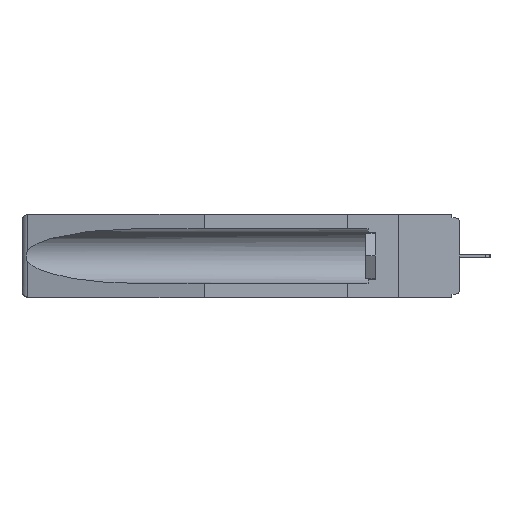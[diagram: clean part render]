
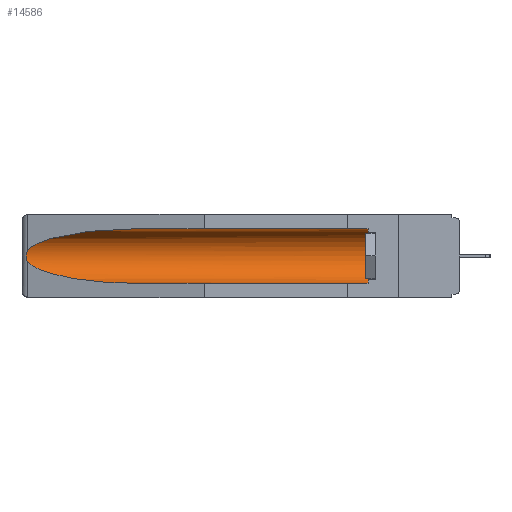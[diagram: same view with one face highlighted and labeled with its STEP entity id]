
A CAD part, left-side view. The second image highlights one B-rep face of the part: STEP entity #14586.
In plain terms, the highlighted cylindrical face has radius 2.857 mm (diameter 5.715 mm), a partial arc.
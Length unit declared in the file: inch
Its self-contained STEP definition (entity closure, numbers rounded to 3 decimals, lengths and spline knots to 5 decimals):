
#298 = EDGE_CURVE ( 'NONE', #9686, #6694, #29425, .T. ) ;
#1093 = AXIS2_PLACEMENT_3D ( 'NONE', #24603, #8456, #6335 ) ;
#1912 = LINE ( 'NONE', #9284, #27571 ) ;
#2595 = AXIS2_PLACEMENT_3D ( 'NONE', #17947, #6588, #8894 ) ;
#3220 = CARTESIAN_POINT ( 'NONE',  ( 0.26597, 1.52961, -0.15275 ) ) ;
#3482 = VERTEX_POINT ( 'NONE', #27198 ) ;
#4576 = CIRCLE ( 'NONE', #2595, 0.1125 ) ;
#4707 =( BOUNDED_CURVE ( )  B_SPLINE_CURVE ( 3, ( #25075, #24777, #6826, #13353 ),
 .UNSPECIFIED., .F., .F. ) 
 B_SPLINE_CURVE_WITH_KNOTS ( ( 4, 4 ),
 ( 4.71239, 6.08839 ),
 .UNSPECIFIED. ) 
 CURVE ( )  GEOMETRIC_REPRESENTATION_ITEM ( )  RATIONAL_B_SPLINE_CURVE ( ( 1., 0.848, 0.848, 1. ) ) 
 REPRESENTATION_ITEM ( '' )  );
#5688 = CARTESIAN_POINT ( 'NONE',  ( 0.26655, 1.53094, -0.18657 ) ) ;
#6335 = DIRECTION ( 'NONE',  ( 0., 0., 1. ) ) ;
#6588 = DIRECTION ( 'NONE',  ( 0., -1., 0. ) ) ;
#6694 = VERTEX_POINT ( 'NONE', #21882 ) ;
#6826 = CARTESIAN_POINT ( 'NONE',  ( 0.25451, 1.48313, -0.09465 ) ) ;
#7929 =( BOUNDED_CURVE ( )  B_SPLINE_CURVE ( 3, ( #25745, #14584, #14305, #14491 ),
 .UNSPECIFIED., .F., .F. ) 
 B_SPLINE_CURVE_WITH_KNOTS ( ( 4, 4 ),
 ( 0.1948, 1.5708 ),
 .UNSPECIFIED. ) 
 CURVE ( )  GEOMETRIC_REPRESENTATION_ITEM ( )  RATIONAL_B_SPLINE_CURVE ( ( 1., 0.848, 0.848, 1. ) ) 
 REPRESENTATION_ITEM ( '' )  );
#8113 = ORIENTED_EDGE ( 'NONE', *, *, #298, .T. ) ;
#8246 = VERTEX_POINT ( 'NONE', #19243 ) ;
#8456 = DIRECTION ( 'NONE',  ( 0., 1., 0. ) ) ;
#8701 = B_SPLINE_CURVE_WITH_KNOTS ( 'NONE', 3,
 ( #23515, #3220, #16812, #16905, #21190, #28296, #10048, #5688, #21302, #14731 ),
 .UNSPECIFIED., .F., .F.,
 ( 4, 2, 2, 2, 4 ),
 ( 0., 0.00029, 0.00058, 0.00087, 0.00117 ),
 .UNSPECIFIED. ) ;
#8894 = DIRECTION ( 'NONE',  ( 0., 0., 1. ) ) ;
#9284 = CARTESIAN_POINT ( 'NONE',  ( 0.155, -0.30754, -0.284 ) ) ;
#9503 = EDGE_CURVE ( 'NONE', #17101, #8246, #8701, .T. ) ;
#9686 = VERTEX_POINT ( 'NONE', #17290 ) ;
#10048 = CARTESIAN_POINT ( 'NONE',  ( 0.2673, 1.53269, -0.17917 ) ) ;
#10454 = FACE_OUTER_BOUND ( 'NONE', #26186, .T. ) ;
#10492 = VECTOR ( 'NONE', #17531, 39.37008 ) ;
#10970 = EDGE_CURVE ( 'NONE', #6694, #17101, #4707, .T. ) ;
#11324 = EDGE_CURVE ( 'NONE', #13011, #9686, #4576, .T. ) ;
#11351 = ORIENTED_EDGE ( 'NONE', *, *, #11324, .T. ) ;
#11894 = DIRECTION ( 'NONE',  ( 0., 1., 0. ) ) ;
#12996 = CARTESIAN_POINT ( 'NONE',  ( 0.155, -0.30754, -0.059 ) ) ;
#13011 = VERTEX_POINT ( 'NONE', #27768 ) ;
#13062 = EDGE_CURVE ( 'NONE', #8246, #3482, #7929, .T. ) ;
#13353 = CARTESIAN_POINT ( 'NONE',  ( 0.26537, 1.52718, -0.14972 ) ) ;
#13440 = ORIENTED_EDGE ( 'NONE', *, *, #9503, .T. ) ;
#14305 = CARTESIAN_POINT ( 'NONE',  ( 0.21114, 1.30732, -0.284 ) ) ;
#14491 = CARTESIAN_POINT ( 'NONE',  ( 0.155, 1.07973, -0.284 ) ) ;
#14584 = CARTESIAN_POINT ( 'NONE',  ( 0.25451, 1.48313, -0.24835 ) ) ;
#14586 = ADVANCED_FACE ( 'NONE', ( #10454 ), #18282, .F. ) ;
#14731 = CARTESIAN_POINT ( 'NONE',  ( 0.26537, 1.52718, -0.19328 ) ) ;
#14808 = EDGE_CURVE ( 'NONE', #13011, #3482, #1912, .T. ) ;
#16812 = CARTESIAN_POINT ( 'NONE',  ( 0.26654, 1.53092, -0.15636 ) ) ;
#16905 = CARTESIAN_POINT ( 'NONE',  ( 0.2673, 1.5327, -0.16383 ) ) ;
#17101 = VERTEX_POINT ( 'NONE', #28718 ) ;
#17290 = CARTESIAN_POINT ( 'NONE',  ( 0.155, 0.126, -0.059 ) ) ;
#17531 = DIRECTION ( 'NONE',  ( 0., 1., 0. ) ) ;
#17947 = CARTESIAN_POINT ( 'NONE',  ( 0.155, 0.126, -0.1715 ) ) ;
#18282 = CYLINDRICAL_SURFACE ( 'NONE', #1093, 0.1125 ) ;
#19243 = CARTESIAN_POINT ( 'NONE',  ( 0.26537, 1.52718, -0.19328 ) ) ;
#21190 = CARTESIAN_POINT ( 'NONE',  ( 0.2675, 1.53308, -0.16763 ) ) ;
#21302 = CARTESIAN_POINT ( 'NONE',  ( 0.26597, 1.5296, -0.19026 ) ) ;
#21882 = CARTESIAN_POINT ( 'NONE',  ( 0.155, 1.07973, -0.059 ) ) ;
#23515 = CARTESIAN_POINT ( 'NONE',  ( 0.26537, 1.52718, -0.14972 ) ) ;
#24603 = CARTESIAN_POINT ( 'NONE',  ( 0.155, -0.30754, -0.1715 ) ) ;
#24777 = CARTESIAN_POINT ( 'NONE',  ( 0.21114, 1.30732, -0.059 ) ) ;
#25075 = CARTESIAN_POINT ( 'NONE',  ( 0.155, 1.07973, -0.059 ) ) ;
#25162 = ORIENTED_EDGE ( 'NONE', *, *, #13062, .T. ) ;
#25284 = ORIENTED_EDGE ( 'NONE', *, *, #10970, .T. ) ;
#25745 = CARTESIAN_POINT ( 'NONE',  ( 0.26537, 1.52718, -0.19328 ) ) ;
#26186 = EDGE_LOOP ( 'NONE', ( #25284, #13440, #25162, #27476, #11351, #8113 ) ) ;
#27198 = CARTESIAN_POINT ( 'NONE',  ( 0.155, 1.07973, -0.284 ) ) ;
#27476 = ORIENTED_EDGE ( 'NONE', *, *, #14808, .F. ) ;
#27571 = VECTOR ( 'NONE', #11894, 39.37008 ) ;
#27768 = CARTESIAN_POINT ( 'NONE',  ( 0.155, 0.126, -0.284 ) ) ;
#28296 = CARTESIAN_POINT ( 'NONE',  ( 0.2675, 1.53308, -0.17534 ) ) ;
#28718 = CARTESIAN_POINT ( 'NONE',  ( 0.26537, 1.52718, -0.14972 ) ) ;
#29425 = LINE ( 'NONE', #12996, #10492 ) ;
